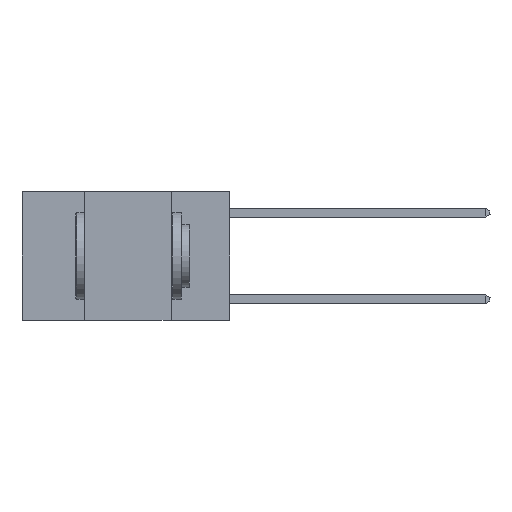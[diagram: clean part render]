
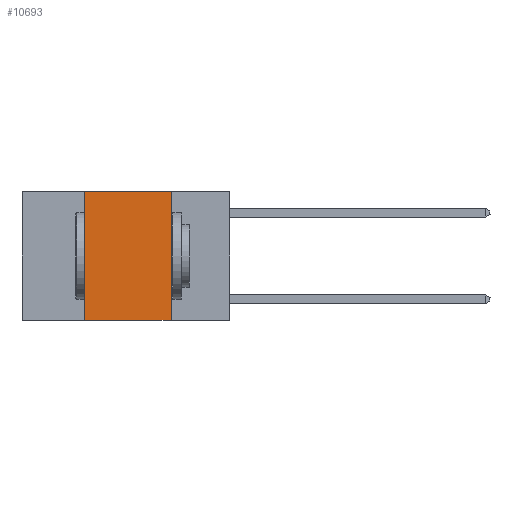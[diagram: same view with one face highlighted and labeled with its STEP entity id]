
A CAD part, left-side view. The second image highlights one B-rep face of the part: STEP entity #10693.
In plain terms, the highlighted planar face has unit normal (-1, 0, 0).
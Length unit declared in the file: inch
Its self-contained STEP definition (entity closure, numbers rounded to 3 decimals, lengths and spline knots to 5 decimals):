
#1133 = EDGE_CURVE ( 'NONE', #14148, #22603, #19114, .T. ) ;
#1198 = CARTESIAN_POINT ( 'NONE',  ( 0., 0.17, 0. ) ) ;
#2102 = CARTESIAN_POINT ( 'NONE',  ( 0., 0.42, 0. ) ) ;
#2695 = EDGE_LOOP ( 'NONE', ( #12356, #13423, #22257, #17868 ) ) ;
#2844 = DIRECTION ( 'NONE',  ( 0., 0., -1. ) ) ;
#4706 = VERTEX_POINT ( 'NONE', #23750 ) ;
#4771 = DIRECTION ( 'NONE',  ( 1., 0., 0. ) ) ;
#4916 = VECTOR ( 'NONE', #12387, 39.37008 ) ;
#5281 = LINE ( 'NONE', #20082, #23371 ) ;
#5599 = EDGE_CURVE ( 'NONE', #4706, #14148, #21611, .T. ) ;
#6341 = VECTOR ( 'NONE', #18979, 39.37008 ) ;
#10612 = DIRECTION ( 'NONE',  ( 0., -1., 0. ) ) ;
#10693 = ADVANCED_FACE ( 'NONE', ( #19801 ), #12045, .F. ) ;
#12045 = PLANE ( 'NONE',  #20147 ) ;
#12193 = CARTESIAN_POINT ( 'NONE',  ( 0., 0.17, 0. ) ) ;
#12356 = ORIENTED_EDGE ( 'NONE', *, *, #1133, .F. ) ;
#12387 = DIRECTION ( 'NONE',  ( 0., -1., 0. ) ) ;
#12646 = CARTESIAN_POINT ( 'NONE',  ( 0., 0.42, -0.37 ) ) ;
#12725 = VECTOR ( 'NONE', #2844, 39.37008 ) ;
#13276 = LINE ( 'NONE', #2102, #6341 ) ;
#13423 = ORIENTED_EDGE ( 'NONE', *, *, #5599, .F. ) ;
#13448 = EDGE_CURVE ( 'NONE', #23829, #22603, #5281, .T. ) ;
#14003 = CARTESIAN_POINT ( 'NONE',  ( 0., 0.6, 0. ) ) ;
#14148 = VERTEX_POINT ( 'NONE', #1198 ) ;
#16156 = CARTESIAN_POINT ( 'NONE',  ( 0., 0.6, 0. ) ) ;
#17127 = EDGE_CURVE ( 'NONE', #23829, #4706, #13276, .T. ) ;
#17868 = ORIENTED_EDGE ( 'NONE', *, *, #13448, .T. ) ;
#18979 = DIRECTION ( 'NONE',  ( 0., 0., 1. ) ) ;
#19114 = LINE ( 'NONE', #12193, #12725 ) ;
#19801 = FACE_OUTER_BOUND ( 'NONE', #2695, .T. ) ;
#20082 = CARTESIAN_POINT ( 'NONE',  ( 0., 0.6, -0.37 ) ) ;
#20130 = CARTESIAN_POINT ( 'NONE',  ( 0., 0.17, -0.37 ) ) ;
#20147 = AXIS2_PLACEMENT_3D ( 'NONE', #14003, #4771, #23469 ) ;
#21611 = LINE ( 'NONE', #16156, #4916 ) ;
#22257 = ORIENTED_EDGE ( 'NONE', *, *, #17127, .F. ) ;
#22603 = VERTEX_POINT ( 'NONE', #20130 ) ;
#23371 = VECTOR ( 'NONE', #10612, 39.37008 ) ;
#23469 = DIRECTION ( 'NONE',  ( 0., 0., -1. ) ) ;
#23750 = CARTESIAN_POINT ( 'NONE',  ( 0., 0.42, 0. ) ) ;
#23829 = VERTEX_POINT ( 'NONE', #12646 ) ;
